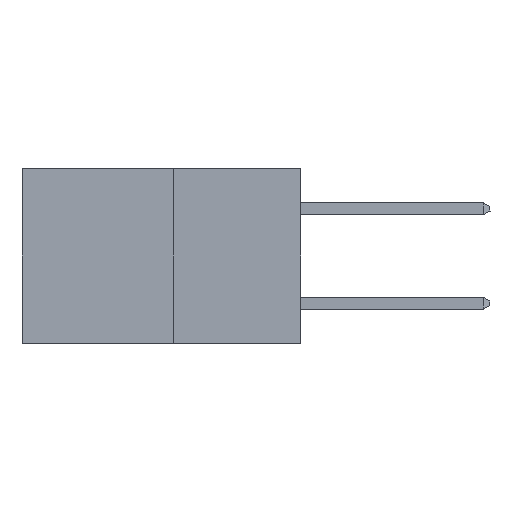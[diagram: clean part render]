
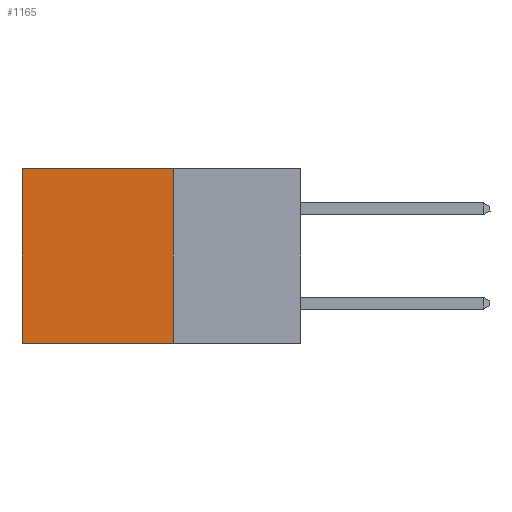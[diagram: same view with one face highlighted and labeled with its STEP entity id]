
A CAD part, left-side view. The second image highlights one B-rep face of the part: STEP entity #1165.
In plain terms, the highlighted planar face has unit normal (-1, 0, 0).
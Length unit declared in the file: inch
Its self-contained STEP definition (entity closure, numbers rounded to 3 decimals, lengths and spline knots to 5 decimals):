
#36 = VERTEX_POINT ( 'NONE', #4941 ) ;
#127 = VERTEX_POINT ( 'NONE', #964 ) ;
#209 = DIRECTION ( 'NONE',  ( 0., 1., 0. ) ) ;
#693 = DIRECTION ( 'NONE',  ( 0., 0., -1. ) ) ;
#842 = CARTESIAN_POINT ( 'NONE',  ( 0.277, 0.27, -0.37 ) ) ;
#948 = DIRECTION ( 'NONE',  ( 0., 0., -1. ) ) ;
#964 = CARTESIAN_POINT ( 'NONE',  ( 0.277, 0.59, -0.37 ) ) ;
#1165 = ADVANCED_FACE ( 'NONE', ( #2042 ), #12103, .F. ) ;
#1357 = VERTEX_POINT ( 'NONE', #5974 ) ;
#1842 = AXIS2_PLACEMENT_3D ( 'NONE', #11579, #8912, #12134 ) ;
#1892 = LINE ( 'NONE', #842, #6772 ) ;
#2042 = FACE_OUTER_BOUND ( 'NONE', #10466, .T. ) ;
#2206 = EDGE_CURVE ( 'NONE', #36, #127, #6324, .T. ) ;
#2807 = CARTESIAN_POINT ( 'NONE',  ( 0.277, 0.59, -0.37 ) ) ;
#2971 = EDGE_CURVE ( 'NONE', #11988, #36, #1892, .T. ) ;
#3073 = EDGE_CURVE ( 'NONE', #11988, #1357, #7195, .T. ) ;
#3096 = ORIENTED_EDGE ( 'NONE', *, *, #5027, .T. ) ;
#3109 = ORIENTED_EDGE ( 'NONE', *, *, #2206, .F. ) ;
#3333 = ORIENTED_EDGE ( 'NONE', *, *, #2971, .F. ) ;
#3424 = ORIENTED_EDGE ( 'NONE', *, *, #3073, .T. ) ;
#3778 = VECTOR ( 'NONE', #6542, 39.37008 ) ;
#4941 = CARTESIAN_POINT ( 'NONE',  ( 0.277, 0.27, -0.37 ) ) ;
#5027 = EDGE_CURVE ( 'NONE', #1357, #127, #9262, .T. ) ;
#5974 = CARTESIAN_POINT ( 'NONE',  ( 0.277, 0.59, 0. ) ) ;
#6324 = LINE ( 'NONE', #6615, #3778 ) ;
#6542 = DIRECTION ( 'NONE',  ( 0., 1., 0. ) ) ;
#6615 = CARTESIAN_POINT ( 'NONE',  ( 0.277, 0.27, -0.37 ) ) ;
#6772 = VECTOR ( 'NONE', #693, 39.37008 ) ;
#7148 = VECTOR ( 'NONE', #948, 39.37008 ) ;
#7195 = LINE ( 'NONE', #12065, #9570 ) ;
#7398 = CARTESIAN_POINT ( 'NONE',  ( 0.277, 0.27, 0. ) ) ;
#8912 = DIRECTION ( 'NONE',  ( 1., 0., 0. ) ) ;
#9262 = LINE ( 'NONE', #2807, #7148 ) ;
#9570 = VECTOR ( 'NONE', #209, 39.37008 ) ;
#10466 = EDGE_LOOP ( 'NONE', ( #3096, #3109, #3333, #3424 ) ) ;
#11579 = CARTESIAN_POINT ( 'NONE',  ( 0.277, 0.27, -0.37 ) ) ;
#11988 = VERTEX_POINT ( 'NONE', #7398 ) ;
#12065 = CARTESIAN_POINT ( 'NONE',  ( 0.277, 0.27, 0. ) ) ;
#12103 = PLANE ( 'NONE',  #1842 ) ;
#12134 = DIRECTION ( 'NONE',  ( 0., 0., -1. ) ) ;
